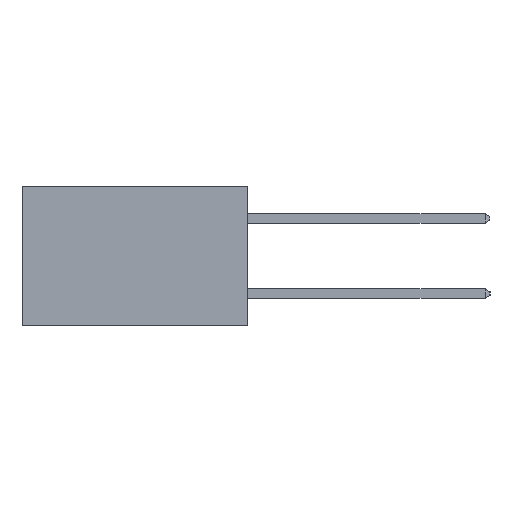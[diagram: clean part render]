
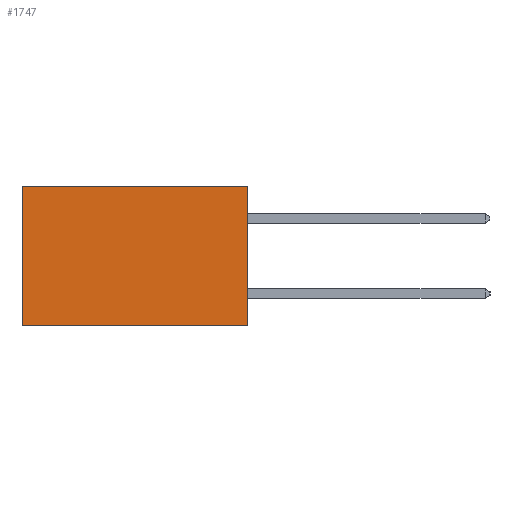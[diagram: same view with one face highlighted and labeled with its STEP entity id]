
A CAD part, left-side view. The second image highlights one B-rep face of the part: STEP entity #1747.
In plain terms, the highlighted planar face has unit normal (-1, 0, 0).
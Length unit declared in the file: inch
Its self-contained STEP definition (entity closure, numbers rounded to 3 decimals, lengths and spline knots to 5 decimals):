
#240 = CARTESIAN_POINT ( 'NONE',  ( 0.2615, 0., -0.37 ) ) ;
#850 = CARTESIAN_POINT ( 'NONE',  ( 0.2615, 0., 0. ) ) ;
#1747 = ADVANCED_FACE ( 'NONE', ( #11893 ), #19785, .F. ) ;
#2247 = DIRECTION ( 'NONE',  ( 0., 1., 0. ) ) ;
#2410 = AXIS2_PLACEMENT_3D ( 'NONE', #18596, #18308, #18339 ) ;
#2879 = DIRECTION ( 'NONE',  ( 0., 1., 0. ) ) ;
#3251 = LINE ( 'NONE', #850, #22356 ) ;
#3272 = LINE ( 'NONE', #240, #17427 ) ;
#4252 = CARTESIAN_POINT ( 'NONE',  ( 0.2615, 0., 0. ) ) ;
#6066 = VECTOR ( 'NONE', #22939, 39.37008 ) ;
#7192 = EDGE_CURVE ( 'NONE', #22201, #7369, #21858, .T. ) ;
#7369 = VERTEX_POINT ( 'NONE', #20178 ) ;
#7385 = VECTOR ( 'NONE', #20371, 39.37008 ) ;
#11070 = CARTESIAN_POINT ( 'NONE',  ( 0.2615, 0., -0.37 ) ) ;
#11893 = FACE_OUTER_BOUND ( 'NONE', #15449, .T. ) ;
#11930 = LINE ( 'NONE', #12895, #7385 ) ;
#12245 = EDGE_CURVE ( 'NONE', #23734, #7369, #3272, .T. ) ;
#12690 = EDGE_CURVE ( 'NONE', #20580, #22201, #3251, .T. ) ;
#12895 = CARTESIAN_POINT ( 'NONE',  ( 0.2615, 0., -0.37 ) ) ;
#13499 = ORIENTED_EDGE ( 'NONE', *, *, #12245, .F. ) ;
#15449 = EDGE_LOOP ( 'NONE', ( #15589, #13499, #20907, #16873 ) ) ;
#15589 = ORIENTED_EDGE ( 'NONE', *, *, #7192, .T. ) ;
#15875 = EDGE_CURVE ( 'NONE', #20580, #23734, #11930, .T. ) ;
#16873 = ORIENTED_EDGE ( 'NONE', *, *, #12690, .T. ) ;
#17427 = VECTOR ( 'NONE', #2247, 39.37008 ) ;
#18308 = DIRECTION ( 'NONE',  ( 1., 0., 0. ) ) ;
#18339 = DIRECTION ( 'NONE',  ( 0., 0., -1. ) ) ;
#18596 = CARTESIAN_POINT ( 'NONE',  ( 0.2615, 0., -0.37 ) ) ;
#19785 = PLANE ( 'NONE',  #2410 ) ;
#20178 = CARTESIAN_POINT ( 'NONE',  ( 0.2615, 0.6, -0.37 ) ) ;
#20371 = DIRECTION ( 'NONE',  ( 0., 0., -1. ) ) ;
#20580 = VERTEX_POINT ( 'NONE', #4252 ) ;
#20907 = ORIENTED_EDGE ( 'NONE', *, *, #15875, .F. ) ;
#21858 = LINE ( 'NONE', #22733, #6066 ) ;
#22201 = VERTEX_POINT ( 'NONE', #23703 ) ;
#22356 = VECTOR ( 'NONE', #2879, 39.37008 ) ;
#22733 = CARTESIAN_POINT ( 'NONE',  ( 0.2615, 0.6, -0.37 ) ) ;
#22939 = DIRECTION ( 'NONE',  ( 0., 0., -1. ) ) ;
#23703 = CARTESIAN_POINT ( 'NONE',  ( 0.2615, 0.6, 0. ) ) ;
#23734 = VERTEX_POINT ( 'NONE', #11070 ) ;
